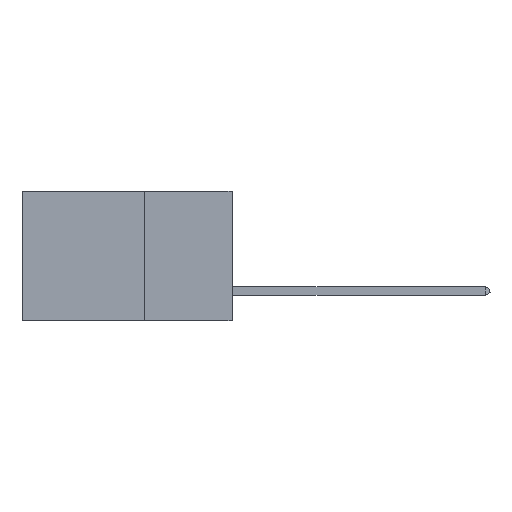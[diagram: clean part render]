
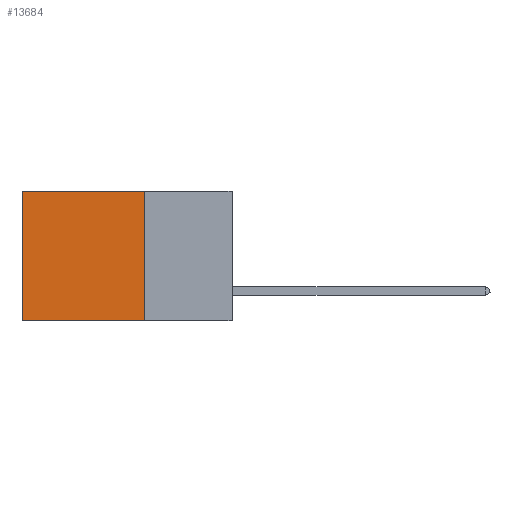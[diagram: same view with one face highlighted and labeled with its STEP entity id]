
A CAD part, left-side view. The second image highlights one B-rep face of the part: STEP entity #13684.
In plain terms, the highlighted planar face has unit normal (-1, 0, 0).
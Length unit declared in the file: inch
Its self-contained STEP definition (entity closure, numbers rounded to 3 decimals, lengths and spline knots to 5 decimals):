
#203 = VERTEX_POINT ( 'NONE', #10822 ) ;
#2413 = CARTESIAN_POINT ( 'NONE',  ( 0.2875, 0.25, 0. ) ) ;
#2853 = ORIENTED_EDGE ( 'NONE', *, *, #6647, .F. ) ;
#4168 = ORIENTED_EDGE ( 'NONE', *, *, #13806, .T. ) ;
#4436 = VECTOR ( 'NONE', #26333, 39.37008 ) ;
#4648 = CARTESIAN_POINT ( 'NONE',  ( 0.2875, 0.25, 0. ) ) ;
#6285 = VECTOR ( 'NONE', #17385, 39.37008 ) ;
#6647 = EDGE_CURVE ( 'NONE', #15565, #17114, #11683, .T. ) ;
#7410 = DIRECTION ( 'NONE',  ( 0., 0., -1. ) ) ;
#8542 = AXIS2_PLACEMENT_3D ( 'NONE', #4648, #15375, #7410 ) ;
#9991 = CARTESIAN_POINT ( 'NONE',  ( 0.2875, 0.25, -0.37 ) ) ;
#10822 = CARTESIAN_POINT ( 'NONE',  ( 0.2875, 0.6, -0.37 ) ) ;
#11683 = LINE ( 'NONE', #2413, #4436 ) ;
#12173 = EDGE_CURVE ( 'NONE', #17114, #203, #34385, .T. ) ;
#13216 = DIRECTION ( 'NONE',  ( 0., 0., -1. ) ) ;
#13684 = ADVANCED_FACE ( 'NONE', ( #34757 ), #28913, .F. ) ;
#13806 = EDGE_CURVE ( 'NONE', #24573, #203, #15153, .T. ) ;
#14890 = CARTESIAN_POINT ( 'NONE',  ( 0.2875, 0.25, 0. ) ) ;
#15153 = LINE ( 'NONE', #32119, #24112 ) ;
#15375 = DIRECTION ( 'NONE',  ( 1., 0., 0. ) ) ;
#15565 = VERTEX_POINT ( 'NONE', #35186 ) ;
#17114 = VERTEX_POINT ( 'NONE', #24867 ) ;
#17332 = VECTOR ( 'NONE', #28761, 39.37008 ) ;
#17385 = DIRECTION ( 'NONE',  ( 0., 1., 0. ) ) ;
#20881 = EDGE_CURVE ( 'NONE', #15565, #24573, #24180, .T. ) ;
#24112 = VECTOR ( 'NONE', #13216, 39.37008 ) ;
#24180 = LINE ( 'NONE', #14890, #6285 ) ;
#24573 = VERTEX_POINT ( 'NONE', #28369 ) ;
#24867 = CARTESIAN_POINT ( 'NONE',  ( 0.2875, 0.25, -0.37 ) ) ;
#26333 = DIRECTION ( 'NONE',  ( 0., 0., -1. ) ) ;
#26720 = ORIENTED_EDGE ( 'NONE', *, *, #12173, .F. ) ;
#28369 = CARTESIAN_POINT ( 'NONE',  ( 0.2875, 0.6, 0. ) ) ;
#28761 = DIRECTION ( 'NONE',  ( 0., 1., 0. ) ) ;
#28913 = PLANE ( 'NONE',  #8542 ) ;
#32119 = CARTESIAN_POINT ( 'NONE',  ( 0.2875, 0.6, 0. ) ) ;
#33895 = ORIENTED_EDGE ( 'NONE', *, *, #20881, .T. ) ;
#34006 = EDGE_LOOP ( 'NONE', ( #4168, #26720, #2853, #33895 ) ) ;
#34385 = LINE ( 'NONE', #9991, #17332 ) ;
#34757 = FACE_OUTER_BOUND ( 'NONE', #34006, .T. ) ;
#35186 = CARTESIAN_POINT ( 'NONE',  ( 0.2875, 0.25, 0. ) ) ;
